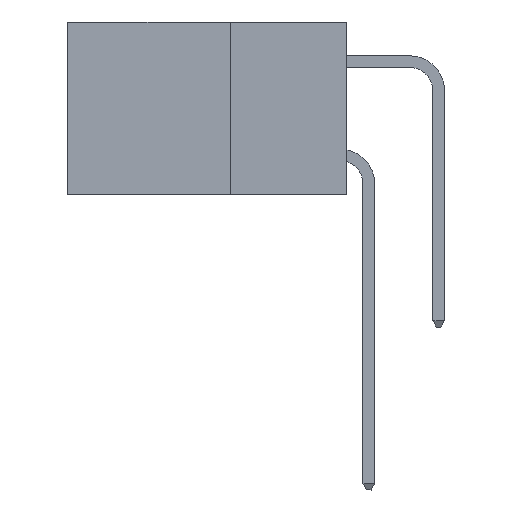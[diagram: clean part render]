
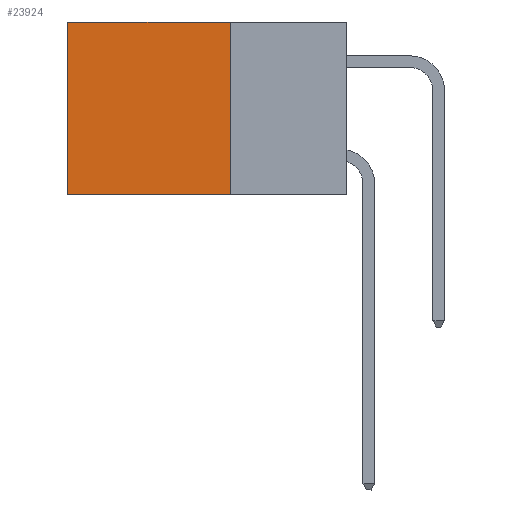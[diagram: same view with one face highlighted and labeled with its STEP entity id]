
A CAD part, left-side view. The second image highlights one B-rep face of the part: STEP entity #23924.
In plain terms, the highlighted planar face has unit normal (-1, 0, 0).
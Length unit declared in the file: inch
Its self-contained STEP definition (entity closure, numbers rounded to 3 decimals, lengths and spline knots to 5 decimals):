
#48 = ORIENTED_EDGE ( 'NONE', *, *, #23467, .T. ) ;
#630 = ORIENTED_EDGE ( 'NONE', *, *, #10602, .T. ) ;
#650 = CARTESIAN_POINT ( 'NONE',  ( 0.2875, 0.25, 0. ) ) ;
#1444 = EDGE_LOOP ( 'NONE', ( #630, #3813, #11957, #48 ) ) ;
#1757 = LINE ( 'NONE', #12724, #11871 ) ;
#1877 = CARTESIAN_POINT ( 'NONE',  ( 0.2875, 0.25, 0. ) ) ;
#2790 = VECTOR ( 'NONE', #23544, 39.37008 ) ;
#3811 = DIRECTION ( 'NONE',  ( 0., 1., 0. ) ) ;
#3813 = ORIENTED_EDGE ( 'NONE', *, *, #22215, .F. ) ;
#4170 = DIRECTION ( 'NONE',  ( 0., 0., -1. ) ) ;
#5588 = DIRECTION ( 'NONE',  ( 0., 0., -1. ) ) ;
#5758 = CARTESIAN_POINT ( 'NONE',  ( 0.2875, 0.6, -0.37 ) ) ;
#5961 = VECTOR ( 'NONE', #20825, 39.37008 ) ;
#6402 = AXIS2_PLACEMENT_3D ( 'NONE', #9494, #22484, #5588 ) ;
#6429 = VERTEX_POINT ( 'NONE', #650 ) ;
#7587 = VERTEX_POINT ( 'NONE', #5758 ) ;
#7677 = FACE_OUTER_BOUND ( 'NONE', #1444, .T. ) ;
#9494 = CARTESIAN_POINT ( 'NONE',  ( 0.2875, 0.25, 0. ) ) ;
#9753 = LINE ( 'NONE', #17299, #5961 ) ;
#10255 = VERTEX_POINT ( 'NONE', #14360 ) ;
#10602 = EDGE_CURVE ( 'NONE', #13491, #7587, #18203, .T. ) ;
#11871 = VECTOR ( 'NONE', #3811, 39.37008 ) ;
#11957 = ORIENTED_EDGE ( 'NONE', *, *, #12520, .F. ) ;
#12503 = CARTESIAN_POINT ( 'NONE',  ( 0.2875, 0.6, 0. ) ) ;
#12520 = EDGE_CURVE ( 'NONE', #6429, #10255, #22423, .T. ) ;
#12724 = CARTESIAN_POINT ( 'NONE',  ( 0.2875, 0.25, 0. ) ) ;
#13491 = VERTEX_POINT ( 'NONE', #22604 ) ;
#14360 = CARTESIAN_POINT ( 'NONE',  ( 0.2875, 0.25, -0.37 ) ) ;
#17299 = CARTESIAN_POINT ( 'NONE',  ( 0.2875, 0.25, -0.37 ) ) ;
#17612 = VECTOR ( 'NONE', #4170, 39.37008 ) ;
#18203 = LINE ( 'NONE', #12503, #2790 ) ;
#20825 = DIRECTION ( 'NONE',  ( 0., 1., 0. ) ) ;
#22128 = PLANE ( 'NONE',  #6402 ) ;
#22215 = EDGE_CURVE ( 'NONE', #10255, #7587, #9753, .T. ) ;
#22423 = LINE ( 'NONE', #1877, #17612 ) ;
#22484 = DIRECTION ( 'NONE',  ( 1., 0., 0. ) ) ;
#22604 = CARTESIAN_POINT ( 'NONE',  ( 0.2875, 0.6, 0. ) ) ;
#23467 = EDGE_CURVE ( 'NONE', #6429, #13491, #1757, .T. ) ;
#23544 = DIRECTION ( 'NONE',  ( 0., 0., -1. ) ) ;
#23924 = ADVANCED_FACE ( 'NONE', ( #7677 ), #22128, .F. ) ;
